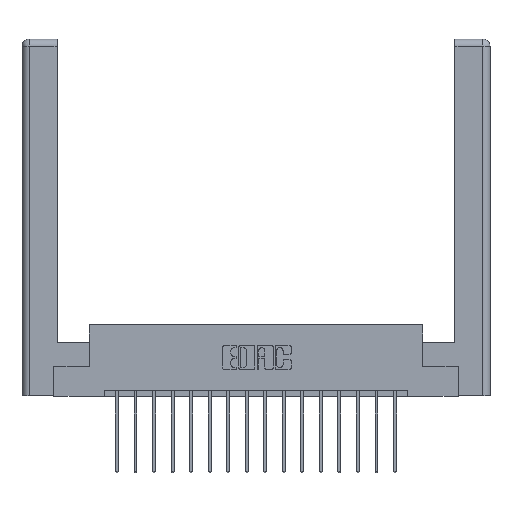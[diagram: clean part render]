
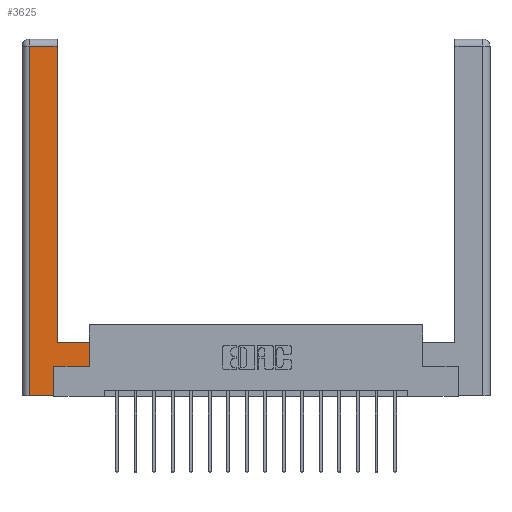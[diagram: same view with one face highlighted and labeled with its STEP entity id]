
A CAD part, top view. The second image highlights one B-rep face of the part: STEP entity #3625.
In plain terms, the highlighted planar face has unit normal (0, 0, 1).
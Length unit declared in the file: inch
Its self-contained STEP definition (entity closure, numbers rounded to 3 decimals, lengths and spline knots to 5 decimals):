
#158 = CARTESIAN_POINT ( 'NONE',  ( 0.0615, 2.94, 0. ) ) ;
#393 = AXIS2_PLACEMENT_3D ( 'NONE', #5005, #10626, #10570 ) ;
#671 = ORIENTED_EDGE ( 'NONE', *, *, #14095, .T. ) ;
#1076 = CARTESIAN_POINT ( 'NONE',  ( 0.295, 0.45, 0. ) ) ;
#1318 = EDGE_LOOP ( 'NONE', ( #14614, #671, #14374, #14912, #10923, #4525, #10994, #7506 ) ) ;
#2297 = LINE ( 'NONE', #9356, #11231 ) ;
#2717 = LINE ( 'NONE', #11742, #6063 ) ;
#2805 = DIRECTION ( 'NONE',  ( 0., -1., 0. ) ) ;
#3293 = CARTESIAN_POINT ( 'NONE',  ( 0.0615, 2.94, 0. ) ) ;
#3625 = ADVANCED_FACE ( 'NONE', ( #16904 ), #16349, .F. ) ;
#3843 = LINE ( 'NONE', #12674, #6087 ) ;
#4033 = VECTOR ( 'NONE', #15642, 39.37008 ) ;
#4310 = DIRECTION ( 'NONE',  ( -1., 0., 0. ) ) ;
#4525 = ORIENTED_EDGE ( 'NONE', *, *, #14345, .T. ) ;
#4730 = VERTEX_POINT ( 'NONE', #16310 ) ;
#5005 = CARTESIAN_POINT ( 'NONE',  ( 0., 0., 0. ) ) ;
#5091 = DIRECTION ( 'NONE',  ( 1., 0., 0. ) ) ;
#5609 = EDGE_CURVE ( 'NONE', #12445, #16441, #8573, .T. ) ;
#5799 = CARTESIAN_POINT ( 'NONE',  ( 0.295, 2.94, 0. ) ) ;
#6063 = VECTOR ( 'NONE', #17445, 39.37008 ) ;
#6084 = CARTESIAN_POINT ( 'NONE',  ( 0.265, 0.245, 0. ) ) ;
#6087 = VECTOR ( 'NONE', #2805, 39.37008 ) ;
#6151 = CARTESIAN_POINT ( 'NONE',  ( 0.0615, 0., 0. ) ) ;
#6624 = DIRECTION ( 'NONE',  ( -1., 0., 0. ) ) ;
#6639 = EDGE_CURVE ( 'NONE', #9643, #12445, #14295, .T. ) ;
#6984 = CARTESIAN_POINT ( 'NONE',  ( 0.295, 3., 0. ) ) ;
#7171 = DIRECTION ( 'NONE',  ( 0., 1., 0. ) ) ;
#7333 = LINE ( 'NONE', #9974, #12689 ) ;
#7506 = ORIENTED_EDGE ( 'NONE', *, *, #5609, .T. ) ;
#7602 = LINE ( 'NONE', #6984, #4033 ) ;
#8528 = LINE ( 'NONE', #158, #18302 ) ;
#8573 = LINE ( 'NONE', #1076, #9250 ) ;
#9250 = VECTOR ( 'NONE', #6624, 39.37008 ) ;
#9356 = CARTESIAN_POINT ( 'NONE',  ( 0.265, 0., 0. ) ) ;
#9643 = VERTEX_POINT ( 'NONE', #9862 ) ;
#9862 = CARTESIAN_POINT ( 'NONE',  ( 0.565, 0.245, 0. ) ) ;
#9974 = CARTESIAN_POINT ( 'NONE',  ( 0.265, 0.245, 0. ) ) ;
#10043 = VECTOR ( 'NONE', #13269, 39.37008 ) ;
#10570 = DIRECTION ( 'NONE',  ( -1., 0., 0. ) ) ;
#10626 = DIRECTION ( 'NONE',  ( 0., 0., -1. ) ) ;
#10923 = ORIENTED_EDGE ( 'NONE', *, *, #15941, .T. ) ;
#10994 = ORIENTED_EDGE ( 'NONE', *, *, #6639, .T. ) ;
#11231 = VECTOR ( 'NONE', #5091, 39.37008 ) ;
#11258 = EDGE_CURVE ( 'NONE', #15050, #16412, #3843, .T. ) ;
#11742 = CARTESIAN_POINT ( 'NONE',  ( 0.565, 0.245, 0. ) ) ;
#12445 = VERTEX_POINT ( 'NONE', #18140 ) ;
#12674 = CARTESIAN_POINT ( 'NONE',  ( 0.0615, 0., 0. ) ) ;
#12689 = VECTOR ( 'NONE', #7171, 39.37008 ) ;
#13034 = CARTESIAN_POINT ( 'NONE',  ( 0.565, 0.45, 0. ) ) ;
#13269 = DIRECTION ( 'NONE',  ( 0., 1., 0. ) ) ;
#13350 = EDGE_CURVE ( 'NONE', #16412, #4730, #2297, .T. ) ;
#14095 = EDGE_CURVE ( 'NONE', #15924, #15050, #8528, .T. ) ;
#14295 = LINE ( 'NONE', #13034, #10043 ) ;
#14345 = EDGE_CURVE ( 'NONE', #15576, #9643, #2717, .T. ) ;
#14374 = ORIENTED_EDGE ( 'NONE', *, *, #11258, .T. ) ;
#14614 = ORIENTED_EDGE ( 'NONE', *, *, #14722, .T. ) ;
#14722 = EDGE_CURVE ( 'NONE', #16441, #15924, #7602, .T. ) ;
#14912 = ORIENTED_EDGE ( 'NONE', *, *, #13350, .T. ) ;
#15050 = VERTEX_POINT ( 'NONE', #3293 ) ;
#15576 = VERTEX_POINT ( 'NONE', #6084 ) ;
#15642 = DIRECTION ( 'NONE',  ( 0., 1., 0. ) ) ;
#15924 = VERTEX_POINT ( 'NONE', #5799 ) ;
#15941 = EDGE_CURVE ( 'NONE', #4730, #15576, #7333, .T. ) ;
#16237 = CARTESIAN_POINT ( 'NONE',  ( 0.295, 0.45, 0. ) ) ;
#16310 = CARTESIAN_POINT ( 'NONE',  ( 0.265, 0., 0. ) ) ;
#16349 = PLANE ( 'NONE',  #393 ) ;
#16412 = VERTEX_POINT ( 'NONE', #6151 ) ;
#16441 = VERTEX_POINT ( 'NONE', #16237 ) ;
#16904 = FACE_OUTER_BOUND ( 'NONE', #1318, .T. ) ;
#17445 = DIRECTION ( 'NONE',  ( 1., 0., 0. ) ) ;
#18140 = CARTESIAN_POINT ( 'NONE',  ( 0.565, 0.45, 0. ) ) ;
#18302 = VECTOR ( 'NONE', #4310, 39.37008 ) ;
